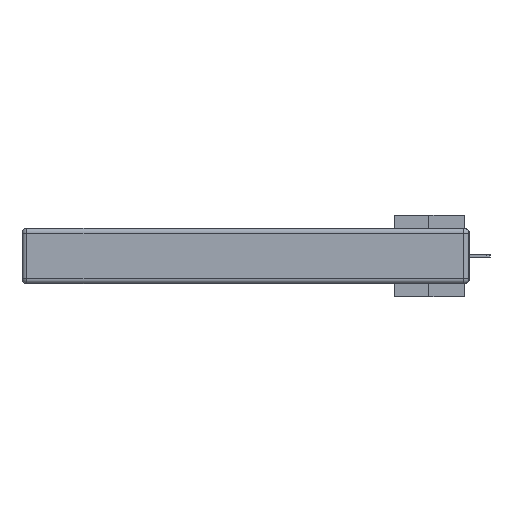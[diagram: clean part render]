
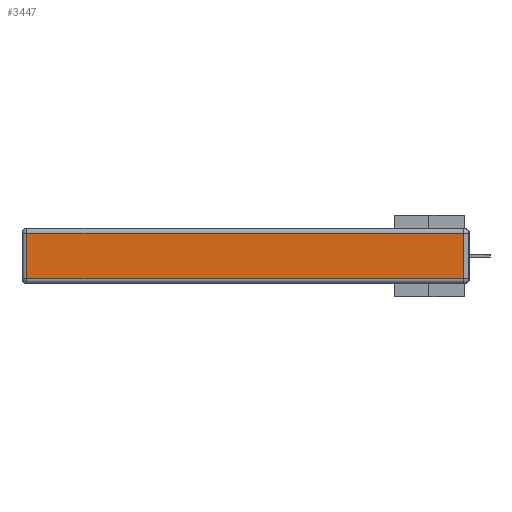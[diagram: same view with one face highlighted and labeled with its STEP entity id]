
A CAD part, left-side view. The second image highlights one B-rep face of the part: STEP entity #3447.
In plain terms, the highlighted planar face has unit normal (-1, 0, 0).
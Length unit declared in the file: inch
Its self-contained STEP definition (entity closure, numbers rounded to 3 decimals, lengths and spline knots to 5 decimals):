
#209 = VECTOR ( 'NONE', #17176, 39.37008 ) ;
#235 = CARTESIAN_POINT ( 'NONE',  ( 0., 2.72, -0.03 ) ) ;
#1246 = DIRECTION ( 'NONE',  ( 0., -1., 0. ) ) ;
#3092 = EDGE_CURVE ( 'NONE', #8295, #14382, #9097, .T. ) ;
#3447 = ADVANCED_FACE ( 'NONE', ( #17846 ), #10113, .T. ) ;
#4157 = CARTESIAN_POINT ( 'NONE',  ( 0., 0., -0.343 ) ) ;
#5018 = CARTESIAN_POINT ( 'NONE',  ( 0., 0.03, -0.343 ) ) ;
#6946 = DIRECTION ( 'NONE',  ( 0., 0., 1. ) ) ;
#8121 = VECTOR ( 'NONE', #18542, 39.37008 ) ;
#8177 = VERTEX_POINT ( 'NONE', #16503 ) ;
#8295 = VERTEX_POINT ( 'NONE', #19128 ) ;
#9078 = LINE ( 'NONE', #20625, #209 ) ;
#9097 = LINE ( 'NONE', #25432, #28183 ) ;
#9207 = VECTOR ( 'NONE', #17849, 39.37008 ) ;
#10113 = PLANE ( 'NONE',  #13500 ) ;
#10362 = CARTESIAN_POINT ( 'NONE',  ( 0., 0.03, -0.313 ) ) ;
#13327 = EDGE_CURVE ( 'NONE', #16714, #8295, #9078, .T. ) ;
#13500 = AXIS2_PLACEMENT_3D ( 'NONE', #4157, #31499, #6946 ) ;
#14382 = VERTEX_POINT ( 'NONE', #10362 ) ;
#16503 = CARTESIAN_POINT ( 'NONE',  ( 0., 0.03, -0.03 ) ) ;
#16714 = VERTEX_POINT ( 'NONE', #235 ) ;
#17176 = DIRECTION ( 'NONE',  ( 0., 0., -1. ) ) ;
#17846 = FACE_OUTER_BOUND ( 'NONE', #18447, .T. ) ;
#17849 = DIRECTION ( 'NONE',  ( 0., 0., 1. ) ) ;
#18447 = EDGE_LOOP ( 'NONE', ( #31838, #20963, #23740, #21074 ) ) ;
#18542 = DIRECTION ( 'NONE',  ( 0., 1., 0. ) ) ;
#19128 = CARTESIAN_POINT ( 'NONE',  ( 0., 2.72, -0.313 ) ) ;
#20315 = LINE ( 'NONE', #5018, #9207 ) ;
#20625 = CARTESIAN_POINT ( 'NONE',  ( 0., 2.72, -0.343 ) ) ;
#20963 = ORIENTED_EDGE ( 'NONE', *, *, #33789, .T. ) ;
#21074 = ORIENTED_EDGE ( 'NONE', *, *, #13327, .T. ) ;
#23740 = ORIENTED_EDGE ( 'NONE', *, *, #33925, .T. ) ;
#24492 = LINE ( 'NONE', #31849, #8121 ) ;
#25432 = CARTESIAN_POINT ( 'NONE',  ( 0., 0., -0.313 ) ) ;
#28183 = VECTOR ( 'NONE', #1246, 39.37008 ) ;
#31499 = DIRECTION ( 'NONE',  ( -1., 0., 0. ) ) ;
#31838 = ORIENTED_EDGE ( 'NONE', *, *, #3092, .T. ) ;
#31849 = CARTESIAN_POINT ( 'NONE',  ( 0., 2.75, -0.03 ) ) ;
#33789 = EDGE_CURVE ( 'NONE', #14382, #8177, #20315, .T. ) ;
#33925 = EDGE_CURVE ( 'NONE', #8177, #16714, #24492, .T. ) ;
